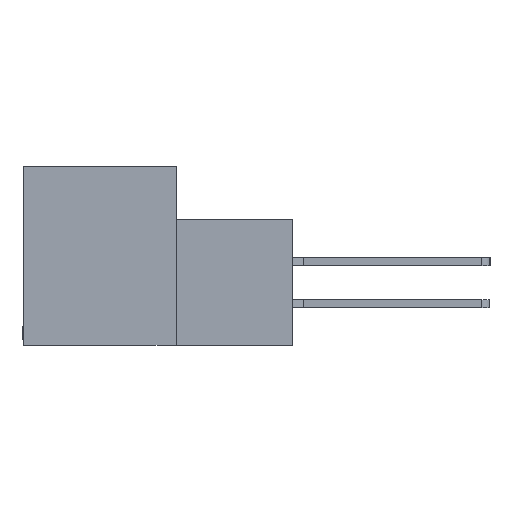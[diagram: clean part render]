
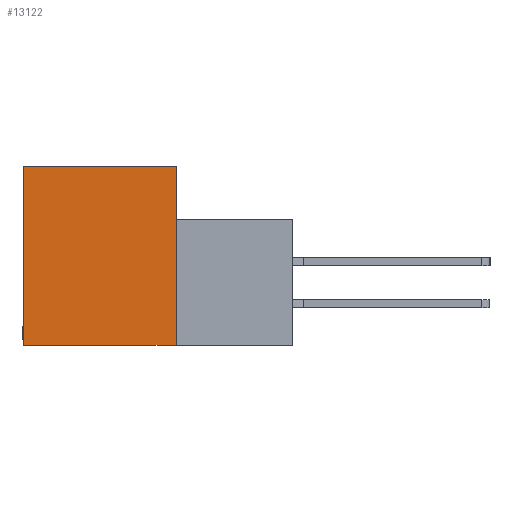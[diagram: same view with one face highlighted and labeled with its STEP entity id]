
A CAD part, left-side view. The second image highlights one B-rep face of the part: STEP entity #13122.
In plain terms, the highlighted planar face has unit normal (-1, 0, 0).
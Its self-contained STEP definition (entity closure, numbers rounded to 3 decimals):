
#145 = CARTESIAN_POINT ( 'NONE',  ( 0., 0., 0. ) ) ;
#1664 = DIRECTION ( 'NONE',  ( 0., 0., -1. ) ) ;
#2434 = DIRECTION ( 'NONE',  ( 0., -1., 0. ) ) ;
#3125 = DIRECTION ( 'NONE',  ( 0., 0., -1. ) ) ;
#3979 = AXIS2_PLACEMENT_3D ( 'NONE', #39274, #17369, #1664 ) ;
#5722 = EDGE_CURVE ( 'NONE', #15184, #25398, #13396, .T. ) ;
#5990 = LINE ( 'NONE', #6767, #14205 ) ;
#6767 = CARTESIAN_POINT ( 'NONE',  ( 0., 11.506, -13.487 ) ) ;
#6911 = EDGE_CURVE ( 'NONE', #9144, #15184, #10396, .T. ) ;
#7041 = VECTOR ( 'NONE', #3125, 1000. ) ;
#9144 = VERTEX_POINT ( 'NONE', #145 ) ;
#10118 = ORIENTED_EDGE ( 'NONE', *, *, #14789, .F. ) ;
#10396 = LINE ( 'NONE', #30670, #7041 ) ;
#10524 = FACE_OUTER_BOUND ( 'NONE', #22092, .T. ) ;
#11250 = ORIENTED_EDGE ( 'NONE', *, *, #35855, .F. ) ;
#11660 = CARTESIAN_POINT ( 'NONE',  ( 0., 11.506, 0. ) ) ;
#13122 = ADVANCED_FACE ( 'NONE', ( #10524 ), #36009, .F. ) ;
#13396 = LINE ( 'NONE', #39342, #33862 ) ;
#13655 = ORIENTED_EDGE ( 'NONE', *, *, #6911, .F. ) ;
#14205 = VECTOR ( 'NONE', #34335, 1000. ) ;
#14789 = EDGE_CURVE ( 'NONE', #20949, #9144, #23041, .T. ) ;
#15184 = VERTEX_POINT ( 'NONE', #29560 ) ;
#17369 = DIRECTION ( 'NONE',  ( 1., 0., 0. ) ) ;
#19385 = CARTESIAN_POINT ( 'NONE',  ( 0., 11.506, -13.487 ) ) ;
#20949 = VERTEX_POINT ( 'NONE', #11660 ) ;
#22092 = EDGE_LOOP ( 'NONE', ( #30587, #13655, #10118, #11250 ) ) ;
#23041 = LINE ( 'NONE', #27549, #39664 ) ;
#25398 = VERTEX_POINT ( 'NONE', #19385 ) ;
#27252 = DIRECTION ( 'NONE',  ( 0., 1., 0. ) ) ;
#27549 = CARTESIAN_POINT ( 'NONE',  ( 0., 11.506, 0. ) ) ;
#29560 = CARTESIAN_POINT ( 'NONE',  ( 0., 0., -13.487 ) ) ;
#30587 = ORIENTED_EDGE ( 'NONE', *, *, #5722, .F. ) ;
#30670 = CARTESIAN_POINT ( 'NONE',  ( 0., 0., 0. ) ) ;
#33862 = VECTOR ( 'NONE', #27252, 1000. ) ;
#34335 = DIRECTION ( 'NONE',  ( 0., 0., 1. ) ) ;
#35855 = EDGE_CURVE ( 'NONE', #25398, #20949, #5990, .T. ) ;
#36009 = PLANE ( 'NONE',  #3979 ) ;
#39274 = CARTESIAN_POINT ( 'NONE',  ( 0., 0., 0. ) ) ;
#39342 = CARTESIAN_POINT ( 'NONE',  ( 0., -8.814, -13.487 ) ) ;
#39664 = VECTOR ( 'NONE', #2434, 1000. ) ;
